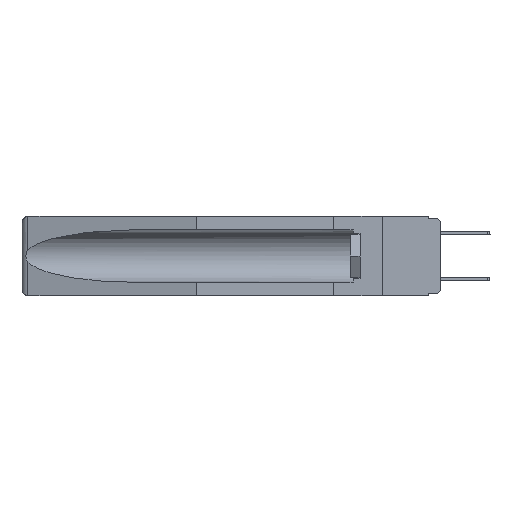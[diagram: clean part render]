
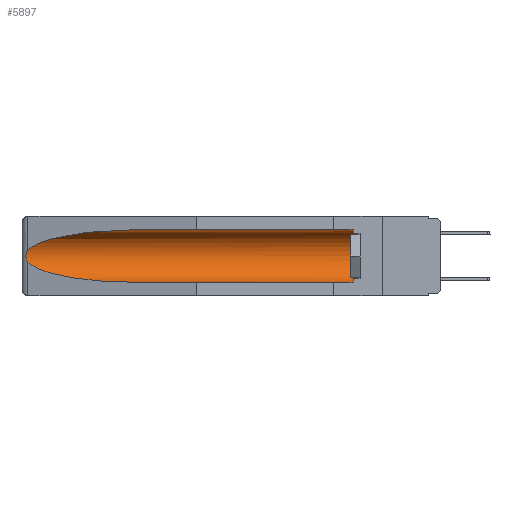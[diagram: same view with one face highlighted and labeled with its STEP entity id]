
A CAD part, left-side view. The second image highlights one B-rep face of the part: STEP entity #5897.
In plain terms, the highlighted cylindrical face has radius 2.857 mm (diameter 5.715 mm), a partial arc.
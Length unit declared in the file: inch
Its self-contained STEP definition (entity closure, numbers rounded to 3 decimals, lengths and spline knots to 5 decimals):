
#309 = CARTESIAN_POINT ( 'NONE',  ( 0.155, 0.126, -0.284 ) ) ;
#414 = DIRECTION ( 'NONE',  ( 0., -1., 0. ) ) ;
#489 = CIRCLE ( 'NONE', #14757, 0.1125 ) ;
#572 = LINE ( 'NONE', #3974, #13083 ) ;
#624 = CARTESIAN_POINT ( 'NONE',  ( 0.26597, 1.5296, -0.19026 ) ) ;
#813 = LINE ( 'NONE', #3557, #10936 ) ;
#1267 = VERTEX_POINT ( 'NONE', #14726 ) ;
#1680 = CARTESIAN_POINT ( 'NONE',  ( 0.2675, 1.53308, -0.16763 ) ) ;
#1724 = CARTESIAN_POINT ( 'NONE',  ( 0.155, 0.126, -0.1715 ) ) ;
#1763 = CARTESIAN_POINT ( 'NONE',  ( 0.26597, 1.52961, -0.15275 ) ) ;
#1776 = CARTESIAN_POINT ( 'NONE',  ( 0.155, 1.07973, -0.284 ) ) ;
#1777 = CARTESIAN_POINT ( 'NONE',  ( 0.26537, 1.52718, -0.14972 ) ) ;
#1827 = EDGE_CURVE ( 'NONE', #5291, #14905, #572, .T. ) ;
#2806 = CARTESIAN_POINT ( 'NONE',  ( 0.2675, 1.53308, -0.17534 ) ) ;
#2818 = CARTESIAN_POINT ( 'NONE',  ( 0.155, 1.07973, -0.059 ) ) ;
#2956 = ORIENTED_EDGE ( 'NONE', *, *, #8004, .T. ) ;
#3259 = ORIENTED_EDGE ( 'NONE', *, *, #15644, .T. ) ;
#3455 = CARTESIAN_POINT ( 'NONE',  ( 0.26537, 1.52718, -0.19328 ) ) ;
#3557 = CARTESIAN_POINT ( 'NONE',  ( 0.155, -0.30754, -0.059 ) ) ;
#3808 = VERTEX_POINT ( 'NONE', #5985 ) ;
#3974 = CARTESIAN_POINT ( 'NONE',  ( 0.155, -0.30754, -0.284 ) ) ;
#4224 = DIRECTION ( 'NONE',  ( 0., 1., 0. ) ) ;
#4286 = CARTESIAN_POINT ( 'NONE',  ( 0.21114, 1.30732, -0.284 ) ) ;
#4584 = DIRECTION ( 'NONE',  ( 0., 0., 1. ) ) ;
#5186 = CARTESIAN_POINT ( 'NONE',  ( 0.155, 1.07973, -0.059 ) ) ;
#5291 = VERTEX_POINT ( 'NONE', #309 ) ;
#5326 = CARTESIAN_POINT ( 'NONE',  ( 0.26537, 1.52718, -0.14972 ) ) ;
#5396 = ORIENTED_EDGE ( 'NONE', *, *, #7139, .T. ) ;
#5578 = CARTESIAN_POINT ( 'NONE',  ( 0.26537, 1.52718, -0.19328 ) ) ;
#5593 = CARTESIAN_POINT ( 'NONE',  ( 0.25451, 1.48313, -0.24835 ) ) ;
#5768 = DIRECTION ( 'NONE',  ( 0., 1., 0. ) ) ;
#5897 = ADVANCED_FACE ( 'NONE', ( #6878 ), #12147, .F. ) ;
#5985 = CARTESIAN_POINT ( 'NONE',  ( 0.155, 0.126, -0.059 ) ) ;
#6246 =( BOUNDED_CURVE ( )  B_SPLINE_CURVE ( 3, ( #15571, #5593, #4286, #1776 ),
 .UNSPECIFIED., .F., .T. ) 
 B_SPLINE_CURVE_WITH_KNOTS ( ( 4, 4 ),
 ( 0.1948, 1.5708 ),
 .UNSPECIFIED. ) 
 CURVE ( )  GEOMETRIC_REPRESENTATION_ITEM ( )  RATIONAL_B_SPLINE_CURVE ( ( 1., 0.848, 0.848, 1. ) ) 
 REPRESENTATION_ITEM ( '' )  );
#6511 = VERTEX_POINT ( 'NONE', #5186 ) ;
#6773 =( BOUNDED_CURVE ( )  B_SPLINE_CURVE ( 3, ( #2818, #8998, #11608, #1777 ),
 .UNSPECIFIED., .F., .T. ) 
 B_SPLINE_CURVE_WITH_KNOTS ( ( 4, 4 ),
 ( 4.71239, 6.08839 ),
 .UNSPECIFIED. ) 
 CURVE ( )  GEOMETRIC_REPRESENTATION_ITEM ( )  RATIONAL_B_SPLINE_CURVE ( ( 1., 0.848, 0.848, 1. ) ) 
 REPRESENTATION_ITEM ( '' )  );
#6878 = FACE_OUTER_BOUND ( 'NONE', #10237, .T. ) ;
#7139 = EDGE_CURVE ( 'NONE', #1267, #14169, #9443, .T. ) ;
#7789 = CARTESIAN_POINT ( 'NONE',  ( 0.2673, 1.53269, -0.17917 ) ) ;
#8004 = EDGE_CURVE ( 'NONE', #5291, #3808, #489, .T. ) ;
#8998 = CARTESIAN_POINT ( 'NONE',  ( 0.21114, 1.30732, -0.059 ) ) ;
#9443 = B_SPLINE_CURVE_WITH_KNOTS ( 'NONE', 3,
 ( #5326, #1763, #13943, #11759, #1680, #2806, #7789, #14100, #624, #5578 ),
 .UNSPECIFIED., .F., .F.,
 ( 4, 2, 2, 2, 4 ),
 ( 0., 0.00029, 0.00058, 0.00087, 0.00117 ),
 .UNSPECIFIED. ) ;
#10237 = EDGE_LOOP ( 'NONE', ( #3259, #5396, #11487, #14484, #2956, #12344 ) ) ;
#10936 = VECTOR ( 'NONE', #5768, 39.37008 ) ;
#11487 = ORIENTED_EDGE ( 'NONE', *, *, #12604, .T. ) ;
#11608 = CARTESIAN_POINT ( 'NONE',  ( 0.25451, 1.48313, -0.09465 ) ) ;
#11759 = CARTESIAN_POINT ( 'NONE',  ( 0.2673, 1.5327, -0.16383 ) ) ;
#12147 = CYLINDRICAL_SURFACE ( 'NONE', #14963, 0.1125 ) ;
#12344 = ORIENTED_EDGE ( 'NONE', *, *, #15414, .T. ) ;
#12604 = EDGE_CURVE ( 'NONE', #14169, #14905, #6246, .T. ) ;
#13083 = VECTOR ( 'NONE', #4224, 39.37008 ) ;
#13943 = CARTESIAN_POINT ( 'NONE',  ( 0.26654, 1.53092, -0.15636 ) ) ;
#14100 = CARTESIAN_POINT ( 'NONE',  ( 0.26655, 1.53094, -0.18657 ) ) ;
#14169 = VERTEX_POINT ( 'NONE', #3455 ) ;
#14335 = CARTESIAN_POINT ( 'NONE',  ( 0.155, -0.30754, -0.1715 ) ) ;
#14484 = ORIENTED_EDGE ( 'NONE', *, *, #1827, .F. ) ;
#14726 = CARTESIAN_POINT ( 'NONE',  ( 0.26537, 1.52718, -0.14972 ) ) ;
#14757 = AXIS2_PLACEMENT_3D ( 'NONE', #1724, #414, #15120 ) ;
#14905 = VERTEX_POINT ( 'NONE', #15921 ) ;
#14963 = AXIS2_PLACEMENT_3D ( 'NONE', #14335, #15634, #4584 ) ;
#15120 = DIRECTION ( 'NONE',  ( 0., 0., 1. ) ) ;
#15414 = EDGE_CURVE ( 'NONE', #3808, #6511, #813, .T. ) ;
#15571 = CARTESIAN_POINT ( 'NONE',  ( 0.26537, 1.52718, -0.19328 ) ) ;
#15634 = DIRECTION ( 'NONE',  ( 0., 1., 0. ) ) ;
#15644 = EDGE_CURVE ( 'NONE', #6511, #1267, #6773, .T. ) ;
#15921 = CARTESIAN_POINT ( 'NONE',  ( 0.155, 1.07973, -0.284 ) ) ;
